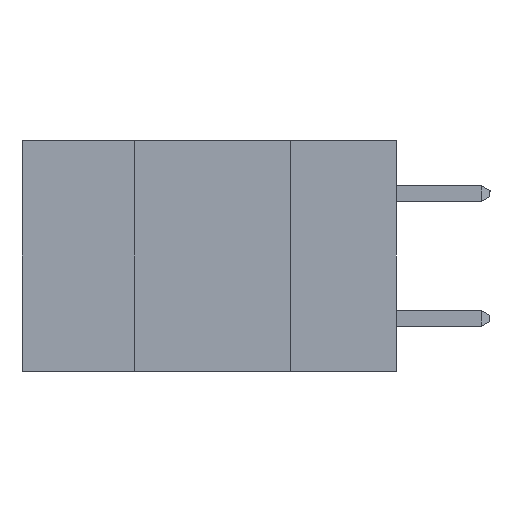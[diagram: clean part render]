
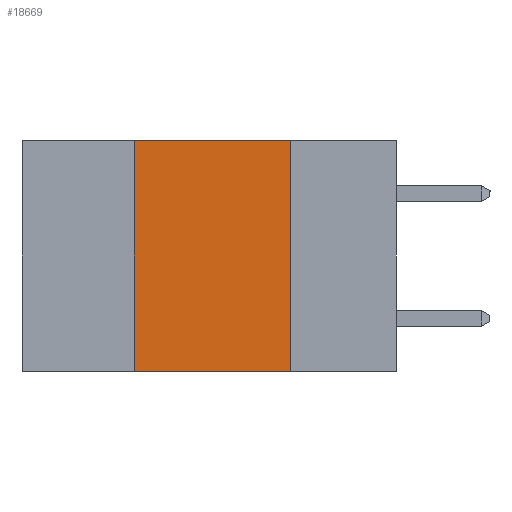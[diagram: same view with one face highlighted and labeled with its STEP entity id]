
A CAD part, left-side view. The second image highlights one B-rep face of the part: STEP entity #18669.
In plain terms, the highlighted planar face has unit normal (-1, 0, 0).
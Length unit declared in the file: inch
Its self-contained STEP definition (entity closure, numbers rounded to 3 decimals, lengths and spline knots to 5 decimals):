
#1342 = LINE ( 'NONE', #3462, #16609 ) ;
#2196 = LINE ( 'NONE', #12265, #8951 ) ;
#2822 = VERTEX_POINT ( 'NONE', #9900 ) ;
#3323 = EDGE_CURVE ( 'NONE', #8544, #15573, #7762, .T. ) ;
#3462 = CARTESIAN_POINT ( 'NONE',  ( 0., 0.17, -0.37 ) ) ;
#5064 = CARTESIAN_POINT ( 'NONE',  ( 0., 0.42, -0.37 ) ) ;
#6183 = DIRECTION ( 'NONE',  ( 0., -1., 0. ) ) ;
#7409 = VECTOR ( 'NONE', #9030, 39.37008 ) ;
#7762 = LINE ( 'NONE', #13824, #25309 ) ;
#8484 = AXIS2_PLACEMENT_3D ( 'NONE', #20184, #9862, #22160 ) ;
#8544 = VERTEX_POINT ( 'NONE', #24887 ) ;
#8951 = VECTOR ( 'NONE', #6183, 39.37008 ) ;
#9030 = DIRECTION ( 'NONE',  ( 0., 0., 1. ) ) ;
#9498 = EDGE_CURVE ( 'NONE', #12822, #15573, #1342, .T. ) ;
#9731 = ORIENTED_EDGE ( 'NONE', *, *, #3323, .T. ) ;
#9862 = DIRECTION ( 'NONE',  ( 1., 0., 0. ) ) ;
#9900 = CARTESIAN_POINT ( 'NONE',  ( 0., 0.42, 0. ) ) ;
#11392 = DIRECTION ( 'NONE',  ( 0., 0., -1. ) ) ;
#12265 = CARTESIAN_POINT ( 'NONE',  ( 0., 0.6, 0. ) ) ;
#12822 = VERTEX_POINT ( 'NONE', #23594 ) ;
#13824 = CARTESIAN_POINT ( 'NONE',  ( 0., 0.6, -0.37 ) ) ;
#14041 = EDGE_CURVE ( 'NONE', #8544, #2822, #14971, .T. ) ;
#14971 = LINE ( 'NONE', #5064, #7409 ) ;
#15573 = VERTEX_POINT ( 'NONE', #16870 ) ;
#16609 = VECTOR ( 'NONE', #11392, 39.37008 ) ;
#16870 = CARTESIAN_POINT ( 'NONE',  ( 0., 0.17, -0.37 ) ) ;
#17482 = EDGE_LOOP ( 'NONE', ( #23708, #21541, #19398, #9731 ) ) ;
#18669 = ADVANCED_FACE ( 'NONE', ( #22028 ), #24029, .F. ) ;
#19398 = ORIENTED_EDGE ( 'NONE', *, *, #14041, .F. ) ;
#19702 = EDGE_CURVE ( 'NONE', #2822, #12822, #2196, .T. ) ;
#19922 = DIRECTION ( 'NONE',  ( 0., -1., 0. ) ) ;
#20184 = CARTESIAN_POINT ( 'NONE',  ( 0., 0.6, 0. ) ) ;
#21541 = ORIENTED_EDGE ( 'NONE', *, *, #19702, .F. ) ;
#22028 = FACE_OUTER_BOUND ( 'NONE', #17482, .T. ) ;
#22160 = DIRECTION ( 'NONE',  ( 0., 0., -1. ) ) ;
#23594 = CARTESIAN_POINT ( 'NONE',  ( 0., 0.17, 0. ) ) ;
#23708 = ORIENTED_EDGE ( 'NONE', *, *, #9498, .F. ) ;
#24029 = PLANE ( 'NONE',  #8484 ) ;
#24887 = CARTESIAN_POINT ( 'NONE',  ( 0., 0.42, -0.37 ) ) ;
#25309 = VECTOR ( 'NONE', #19922, 39.37008 ) ;
